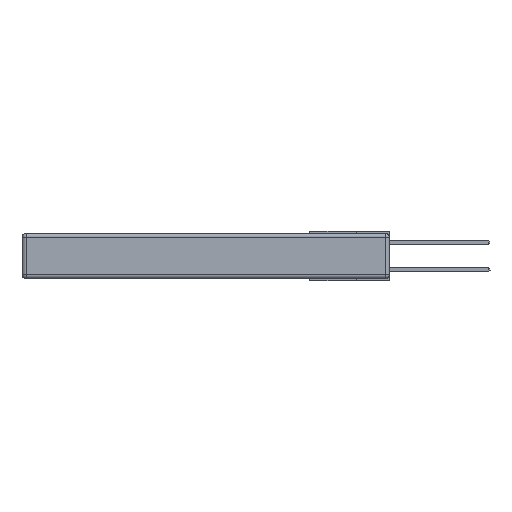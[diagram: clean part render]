
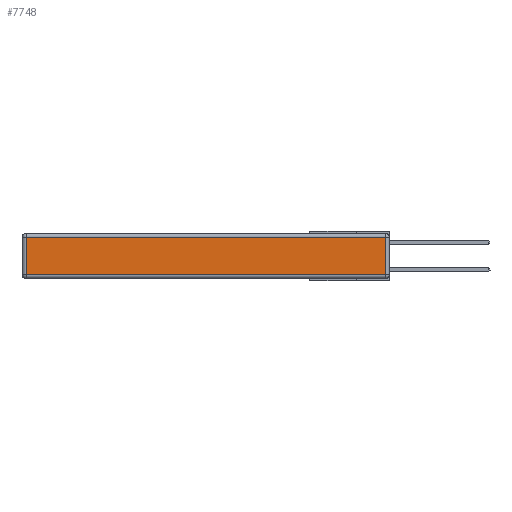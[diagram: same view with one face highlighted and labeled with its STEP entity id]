
A CAD part, left-side view. The second image highlights one B-rep face of the part: STEP entity #7748.
In plain terms, the highlighted planar face has unit normal (-1, 0, 0).
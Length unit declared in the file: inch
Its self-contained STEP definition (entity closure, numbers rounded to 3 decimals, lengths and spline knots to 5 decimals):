
#251 = PLANE ( 'NONE',  #4332 ) ;
#264 = CARTESIAN_POINT ( 'NONE',  ( 0., 2.72, -0.03 ) ) ;
#301 = CARTESIAN_POINT ( 'NONE',  ( 0., 2.75, -0.03 ) ) ;
#1625 = DIRECTION ( 'NONE',  ( -1., 0., 0. ) ) ;
#1871 = DIRECTION ( 'NONE',  ( 0., 1., 0. ) ) ;
#2360 = VECTOR ( 'NONE', #1871, 39.37008 ) ;
#3068 = LINE ( 'NONE', #3432, #13923 ) ;
#3191 = ORIENTED_EDGE ( 'NONE', *, *, #15022, .T. ) ;
#3432 = CARTESIAN_POINT ( 'NONE',  ( 0., 0., -0.313 ) ) ;
#4332 = AXIS2_PLACEMENT_3D ( 'NONE', #5722, #1625, #10416 ) ;
#4467 = EDGE_CURVE ( 'NONE', #10063, #17304, #16102, .T. ) ;
#4777 = VECTOR ( 'NONE', #16596, 39.37008 ) ;
#5716 = ORIENTED_EDGE ( 'NONE', *, *, #10590, .T. ) ;
#5722 = CARTESIAN_POINT ( 'NONE',  ( 0., 0., -0.343 ) ) ;
#6335 = LINE ( 'NONE', #15190, #4777 ) ;
#7110 = FACE_OUTER_BOUND ( 'NONE', #16755, .T. ) ;
#7155 = ORIENTED_EDGE ( 'NONE', *, *, #4467, .T. ) ;
#7189 = CARTESIAN_POINT ( 'NONE',  ( 0., 0.03, -0.343 ) ) ;
#7526 = LINE ( 'NONE', #7189, #10392 ) ;
#7748 = ADVANCED_FACE ( 'NONE', ( #7110 ), #251, .T. ) ;
#8932 = EDGE_CURVE ( 'NONE', #16198, #10063, #7526, .T. ) ;
#10063 = VERTEX_POINT ( 'NONE', #15293 ) ;
#10392 = VECTOR ( 'NONE', #14309, 39.37008 ) ;
#10416 = DIRECTION ( 'NONE',  ( 0., 0., 1. ) ) ;
#10590 = EDGE_CURVE ( 'NONE', #17304, #16641, #6335, .T. ) ;
#13923 = VECTOR ( 'NONE', #17748, 39.37008 ) ;
#14309 = DIRECTION ( 'NONE',  ( 0., 0., 1. ) ) ;
#15022 = EDGE_CURVE ( 'NONE', #16641, #16198, #3068, .T. ) ;
#15190 = CARTESIAN_POINT ( 'NONE',  ( 0., 2.72, -0.343 ) ) ;
#15293 = CARTESIAN_POINT ( 'NONE',  ( 0., 0.03, -0.03 ) ) ;
#15686 = CARTESIAN_POINT ( 'NONE',  ( 0., 0.03, -0.313 ) ) ;
#16102 = LINE ( 'NONE', #301, #2360 ) ;
#16198 = VERTEX_POINT ( 'NONE', #15686 ) ;
#16596 = DIRECTION ( 'NONE',  ( 0., 0., -1. ) ) ;
#16641 = VERTEX_POINT ( 'NONE', #18327 ) ;
#16755 = EDGE_LOOP ( 'NONE', ( #3191, #18314, #7155, #5716 ) ) ;
#17304 = VERTEX_POINT ( 'NONE', #264 ) ;
#17748 = DIRECTION ( 'NONE',  ( 0., -1., 0. ) ) ;
#18314 = ORIENTED_EDGE ( 'NONE', *, *, #8932, .T. ) ;
#18327 = CARTESIAN_POINT ( 'NONE',  ( 0., 2.72, -0.313 ) ) ;
